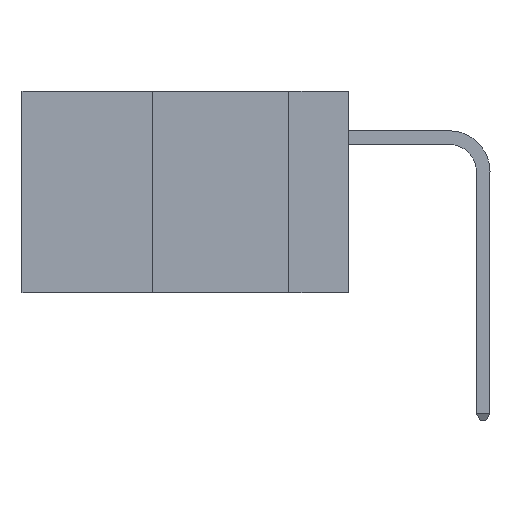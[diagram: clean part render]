
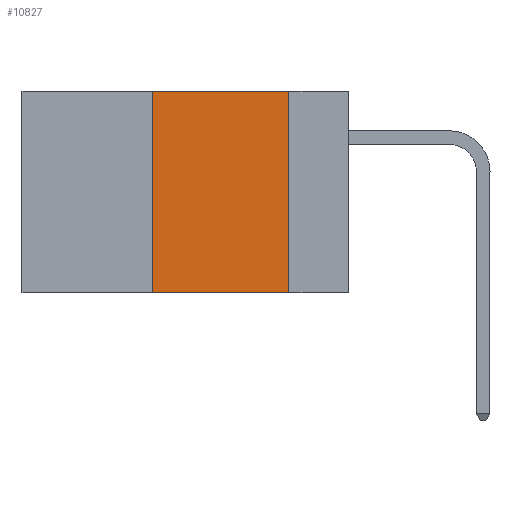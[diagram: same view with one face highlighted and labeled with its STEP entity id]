
A CAD part, left-side view. The second image highlights one B-rep face of the part: STEP entity #10827.
In plain terms, the highlighted planar face has unit normal (-1, 0, 0).
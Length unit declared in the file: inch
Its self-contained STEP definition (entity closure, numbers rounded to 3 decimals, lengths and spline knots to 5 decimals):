
#1691 = PLANE ( 'NONE',  #13006 ) ;
#2290 = LINE ( 'NONE', #14471, #5160 ) ;
#2425 = DIRECTION ( 'NONE',  ( 0., -1., 0. ) ) ;
#2633 = CARTESIAN_POINT ( 'NONE',  ( 0., 0.36, 0. ) ) ;
#2885 = CARTESIAN_POINT ( 'NONE',  ( 0., 0.11, 0. ) ) ;
#2943 = DIRECTION ( 'NONE',  ( 0., 0., -1. ) ) ;
#3568 = LINE ( 'NONE', #2885, #12850 ) ;
#3574 = EDGE_CURVE ( 'NONE', #5038, #6623, #8380, .T. ) ;
#3742 = ORIENTED_EDGE ( 'NONE', *, *, #8227, .F. ) ;
#3834 = CARTESIAN_POINT ( 'NONE',  ( 0., 0.36, 0. ) ) ;
#5038 = VERTEX_POINT ( 'NONE', #3834 ) ;
#5160 = VECTOR ( 'NONE', #2425, 39.37008 ) ;
#5242 = CARTESIAN_POINT ( 'NONE',  ( 0., 0.11, -0.37 ) ) ;
#5599 = FACE_OUTER_BOUND ( 'NONE', #11658, .T. ) ;
#6071 = CARTESIAN_POINT ( 'NONE',  ( 0., 0.6, 0. ) ) ;
#6346 = DIRECTION ( 'NONE',  ( 0., 0., 1. ) ) ;
#6623 = VERTEX_POINT ( 'NONE', #13454 ) ;
#6977 = ORIENTED_EDGE ( 'NONE', *, *, #3574, .F. ) ;
#7297 = DIRECTION ( 'NONE',  ( 0., -1., 0. ) ) ;
#7774 = ORIENTED_EDGE ( 'NONE', *, *, #14913, .T. ) ;
#7929 = EDGE_CURVE ( 'NONE', #6623, #15098, #3568, .T. ) ;
#8227 = EDGE_CURVE ( 'NONE', #12113, #5038, #13025, .T. ) ;
#8380 = LINE ( 'NONE', #6071, #14719 ) ;
#9099 = VECTOR ( 'NONE', #6346, 39.37008 ) ;
#10230 = DIRECTION ( 'NONE',  ( 1., 0., 0. ) ) ;
#10827 = ADVANCED_FACE ( 'NONE', ( #5599 ), #1691, .F. ) ;
#11658 = EDGE_LOOP ( 'NONE', ( #12589, #6977, #3742, #7774 ) ) ;
#12113 = VERTEX_POINT ( 'NONE', #12605 ) ;
#12589 = ORIENTED_EDGE ( 'NONE', *, *, #7929, .F. ) ;
#12592 = DIRECTION ( 'NONE',  ( 0., 0., -1. ) ) ;
#12605 = CARTESIAN_POINT ( 'NONE',  ( 0., 0.36, -0.37 ) ) ;
#12850 = VECTOR ( 'NONE', #12592, 39.37008 ) ;
#13006 = AXIS2_PLACEMENT_3D ( 'NONE', #14961, #10230, #2943 ) ;
#13025 = LINE ( 'NONE', #2633, #9099 ) ;
#13454 = CARTESIAN_POINT ( 'NONE',  ( 0., 0.11, 0. ) ) ;
#14471 = CARTESIAN_POINT ( 'NONE',  ( 0., 0.6, -0.37 ) ) ;
#14719 = VECTOR ( 'NONE', #7297, 39.37008 ) ;
#14913 = EDGE_CURVE ( 'NONE', #12113, #15098, #2290, .T. ) ;
#14961 = CARTESIAN_POINT ( 'NONE',  ( 0., 0.6, 0. ) ) ;
#15098 = VERTEX_POINT ( 'NONE', #5242 ) ;
